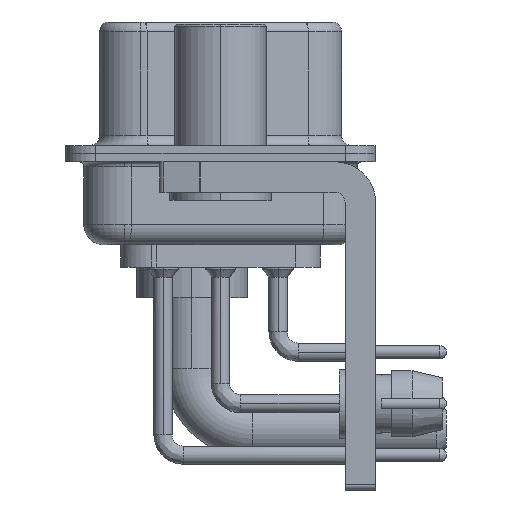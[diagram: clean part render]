
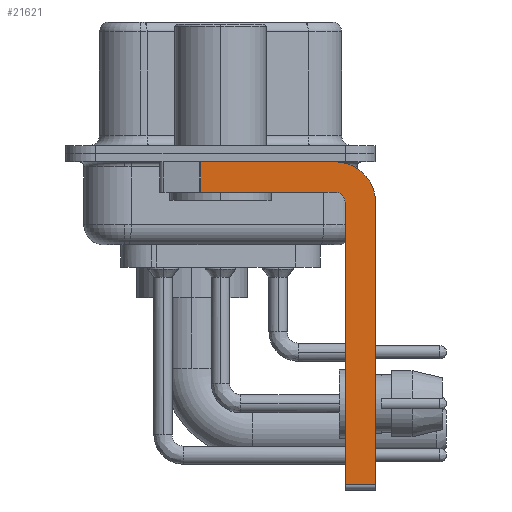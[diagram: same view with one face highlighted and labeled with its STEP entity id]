
A CAD part, left-side view. The second image highlights one B-rep face of the part: STEP entity #21621.
In plain terms, the highlighted planar face has unit normal (-1, 0, 0).
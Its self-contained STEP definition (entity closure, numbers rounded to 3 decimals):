
#152 = DIRECTION ( 'NONE',  ( 0., -1., 0. ) ) ;
#479 = CARTESIAN_POINT ( 'NONE',  ( -2.9, 0.978, -1.9 ) ) ;
#1636 = VECTOR ( 'NONE', #152, 1000. ) ;
#1668 = FACE_OUTER_BOUND ( 'NONE', #16842, .T. ) ;
#1857 = EDGE_CURVE ( 'NONE', #8055, #6235, #16622, .T. ) ;
#3382 = VERTEX_POINT ( 'NONE', #10990 ) ;
#4041 = DIRECTION ( 'NONE',  ( 0., 0., -1. ) ) ;
#4595 = VERTEX_POINT ( 'NONE', #15339 ) ;
#4919 = CARTESIAN_POINT ( 'NONE',  ( -2.9, -5.65, -2.4 ) ) ;
#5307 = CARTESIAN_POINT ( 'NONE',  ( -2.9, -6.15, -16.6 ) ) ;
#5391 = VERTEX_POINT ( 'NONE', #26844 ) ;
#6235 = VERTEX_POINT ( 'NONE', #24428 ) ;
#6391 = EDGE_CURVE ( 'NONE', #4595, #6235, #25632, .T. ) ;
#6540 = CIRCLE ( 'NONE', #37622, 0.5 ) ;
#8016 = DIRECTION ( 'NONE',  ( 0., 0., 1. ) ) ;
#8055 = VERTEX_POINT ( 'NONE', #21952 ) ;
#9234 = VERTEX_POINT ( 'NONE', #19371 ) ;
#9727 = VERTEX_POINT ( 'NONE', #36037 ) ;
#9935 = EDGE_CURVE ( 'NONE', #8055, #18553, #19632, .T. ) ;
#10238 = CARTESIAN_POINT ( 'NONE',  ( -2.9, -5.65, -2.4 ) ) ;
#10990 = CARTESIAN_POINT ( 'NONE',  ( -2.9, -6.15, -2.4 ) ) ;
#11161 = PLANE ( 'NONE',  #33603 ) ;
#11268 = CARTESIAN_POINT ( 'NONE',  ( -2.9, -5.65, -0.4 ) ) ;
#11356 = DIRECTION ( 'NONE',  ( 1., 0., 0. ) ) ;
#15339 = CARTESIAN_POINT ( 'NONE',  ( -2.9, -5.65, -1.9 ) ) ;
#15443 = CARTESIAN_POINT ( 'NONE',  ( -2.9, -5.65, -16.35 ) ) ;
#16019 = AXIS2_PLACEMENT_3D ( 'NONE', #10238, #19217, #4041 ) ;
#16417 = DIRECTION ( 'NONE',  ( 0., 0., -1. ) ) ;
#16622 = LINE ( 'NONE', #479, #26273 ) ;
#16705 = EDGE_CURVE ( 'NONE', #3382, #4595, #6540, .T. ) ;
#16842 = EDGE_LOOP ( 'NONE', ( #29516, #29391, #29247, #35973, #40215, #29738, #18831, #17249 ) ) ;
#17173 = DIRECTION ( 'NONE',  ( -1., 0., 0. ) ) ;
#17249 = ORIENTED_EDGE ( 'NONE', *, *, #28223, .F. ) ;
#18553 = VERTEX_POINT ( 'NONE', #11268 ) ;
#18831 = ORIENTED_EDGE ( 'NONE', *, *, #24478, .F. ) ;
#19217 = DIRECTION ( 'NONE',  ( 1., 0., 0. ) ) ;
#19371 = CARTESIAN_POINT ( 'NONE',  ( -2.9, -6.15, -16.35 ) ) ;
#19632 = LINE ( 'NONE', #28490, #1636 ) ;
#21021 = DIRECTION ( 'NONE',  ( 0., 0., -1. ) ) ;
#21621 = ADVANCED_FACE ( 'NONE', ( #1668 ), #11161, .F. ) ;
#21884 = DIRECTION ( 'NONE',  ( 0., -1., 0. ) ) ;
#21952 = CARTESIAN_POINT ( 'NONE',  ( -2.9, 0.978, -0.4 ) ) ;
#23508 = LINE ( 'NONE', #33203, #25123 ) ;
#23789 = VECTOR ( 'NONE', #21884, 1000. ) ;
#24428 = CARTESIAN_POINT ( 'NONE',  ( -2.9, 0.978, -1.9 ) ) ;
#24478 = EDGE_CURVE ( 'NONE', #5391, #9727, #23508, .T. ) ;
#25123 = VECTOR ( 'NONE', #21021, 1000. ) ;
#25632 = LINE ( 'NONE', #34766, #29801 ) ;
#26273 = VECTOR ( 'NONE', #16417, 1000. ) ;
#26844 = CARTESIAN_POINT ( 'NONE',  ( -2.9, -7.65, -2.4 ) ) ;
#27310 = DIRECTION ( 'NONE',  ( 0., 0., -1. ) ) ;
#28223 = EDGE_CURVE ( 'NONE', #18553, #5391, #37173, .T. ) ;
#28293 = EDGE_CURVE ( 'NONE', #9234, #3382, #36383, .T. ) ;
#28490 = CARTESIAN_POINT ( 'NONE',  ( -2.9, 3., -0.4 ) ) ;
#28597 = VECTOR ( 'NONE', #30559, 1000. ) ;
#29247 = ORIENTED_EDGE ( 'NONE', *, *, #6391, .F. ) ;
#29391 = ORIENTED_EDGE ( 'NONE', *, *, #1857, .T. ) ;
#29436 = LINE ( 'NONE', #15443, #23789 ) ;
#29516 = ORIENTED_EDGE ( 'NONE', *, *, #9935, .F. ) ;
#29738 = ORIENTED_EDGE ( 'NONE', *, *, #33984, .T. ) ;
#29801 = VECTOR ( 'NONE', #37670, 1000. ) ;
#30418 = CARTESIAN_POINT ( 'NONE',  ( -2.9, -5.65, -2.4 ) ) ;
#30559 = DIRECTION ( 'NONE',  ( 0., 0., 1. ) ) ;
#33203 = CARTESIAN_POINT ( 'NONE',  ( -2.9, -7.65, -2.4 ) ) ;
#33603 = AXIS2_PLACEMENT_3D ( 'NONE', #30418, #11356, #27310 ) ;
#33984 = EDGE_CURVE ( 'NONE', #9234, #9727, #29436, .T. ) ;
#34766 = CARTESIAN_POINT ( 'NONE',  ( -2.9, -5.65, -1.9 ) ) ;
#35973 = ORIENTED_EDGE ( 'NONE', *, *, #16705, .F. ) ;
#36037 = CARTESIAN_POINT ( 'NONE',  ( -2.9, -7.65, -16.35 ) ) ;
#36383 = LINE ( 'NONE', #5307, #28597 ) ;
#37173 = CIRCLE ( 'NONE', #16019, 2. ) ;
#37622 = AXIS2_PLACEMENT_3D ( 'NONE', #4919, #17173, #8016 ) ;
#37670 = DIRECTION ( 'NONE',  ( 0., 1., 0. ) ) ;
#40215 = ORIENTED_EDGE ( 'NONE', *, *, #28293, .F. ) ;
